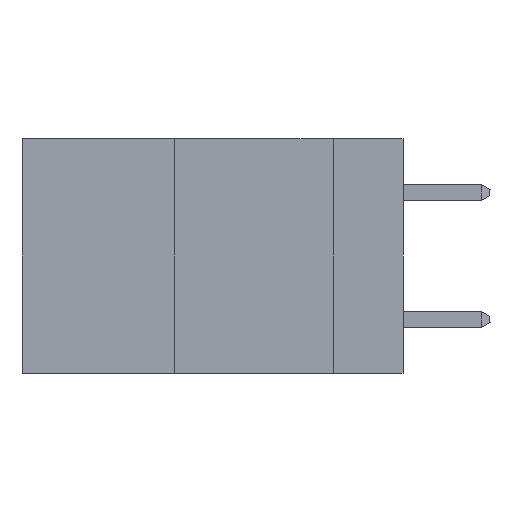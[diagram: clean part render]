
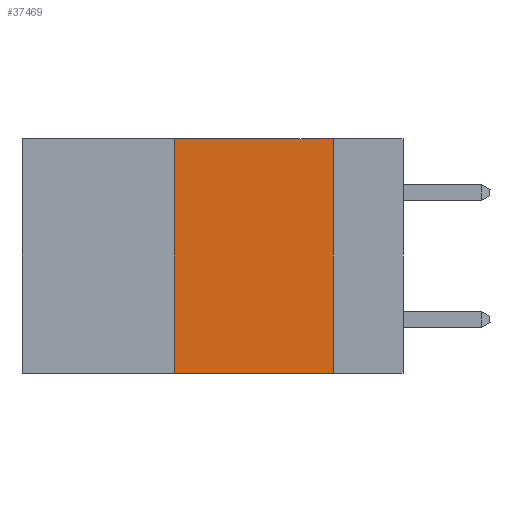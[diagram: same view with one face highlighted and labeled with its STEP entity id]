
A CAD part, left-side view. The second image highlights one B-rep face of the part: STEP entity #37469.
In plain terms, the highlighted planar face has unit normal (-1, 0, 0).
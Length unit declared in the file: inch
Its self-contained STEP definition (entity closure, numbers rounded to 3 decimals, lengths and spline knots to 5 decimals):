
#3783 = CARTESIAN_POINT ( 'NONE',  ( 0., 0.36, 0. ) ) ;
#3951 = CARTESIAN_POINT ( 'NONE',  ( 0., 0.11, -0.37 ) ) ;
#4002 = ORIENTED_EDGE ( 'NONE', *, *, #43798, .F. ) ;
#4922 = LINE ( 'NONE', #14007, #24656 ) ;
#6808 = EDGE_CURVE ( 'NONE', #44418, #27941, #8070, .T. ) ;
#8070 = LINE ( 'NONE', #25759, #14203 ) ;
#11955 = EDGE_LOOP ( 'NONE', ( #22736, #4002, #26385, #15980 ) ) ;
#13514 = EDGE_CURVE ( 'NONE', #21365, #27941, #41792, .T. ) ;
#14007 = CARTESIAN_POINT ( 'NONE',  ( 0., 0.6, 0. ) ) ;
#14203 = VECTOR ( 'NONE', #14848, 39.37008 ) ;
#14848 = DIRECTION ( 'NONE',  ( 0., -1., 0. ) ) ;
#15980 = ORIENTED_EDGE ( 'NONE', *, *, #6808, .T. ) ;
#17426 = LINE ( 'NONE', #3783, #38407 ) ;
#19065 = CARTESIAN_POINT ( 'NONE',  ( 0., 0.36, 0. ) ) ;
#19125 = DIRECTION ( 'NONE',  ( 0., 0., -1. ) ) ;
#19638 = FACE_OUTER_BOUND ( 'NONE', #11955, .T. ) ;
#21365 = VERTEX_POINT ( 'NONE', #30137 ) ;
#21453 = PLANE ( 'NONE',  #44649 ) ;
#22736 = ORIENTED_EDGE ( 'NONE', *, *, #13514, .F. ) ;
#24412 = DIRECTION ( 'NONE',  ( 0., -1., 0. ) ) ;
#24656 = VECTOR ( 'NONE', #24412, 39.37008 ) ;
#24786 = DIRECTION ( 'NONE',  ( 1., 0., 0. ) ) ;
#25759 = CARTESIAN_POINT ( 'NONE',  ( 0., 0.6, -0.37 ) ) ;
#26385 = ORIENTED_EDGE ( 'NONE', *, *, #42414, .F. ) ;
#27941 = VERTEX_POINT ( 'NONE', #3951 ) ;
#30137 = CARTESIAN_POINT ( 'NONE',  ( 0., 0.11, 0. ) ) ;
#32183 = VECTOR ( 'NONE', #19125, 39.37008 ) ;
#32187 = DIRECTION ( 'NONE',  ( 0., 0., 1. ) ) ;
#32824 = VERTEX_POINT ( 'NONE', #19065 ) ;
#35256 = CARTESIAN_POINT ( 'NONE',  ( 0., 0.36, -0.37 ) ) ;
#35530 = CARTESIAN_POINT ( 'NONE',  ( 0., 0.6, 0. ) ) ;
#36973 = CARTESIAN_POINT ( 'NONE',  ( 0., 0.11, 0. ) ) ;
#37469 = ADVANCED_FACE ( 'NONE', ( #19638 ), #21453, .F. ) ;
#38407 = VECTOR ( 'NONE', #32187, 39.37008 ) ;
#38861 = DIRECTION ( 'NONE',  ( 0., 0., -1. ) ) ;
#41792 = LINE ( 'NONE', #36973, #32183 ) ;
#42414 = EDGE_CURVE ( 'NONE', #44418, #32824, #17426, .T. ) ;
#43798 = EDGE_CURVE ( 'NONE', #32824, #21365, #4922, .T. ) ;
#44418 = VERTEX_POINT ( 'NONE', #35256 ) ;
#44649 = AXIS2_PLACEMENT_3D ( 'NONE', #35530, #24786, #38861 ) ;
